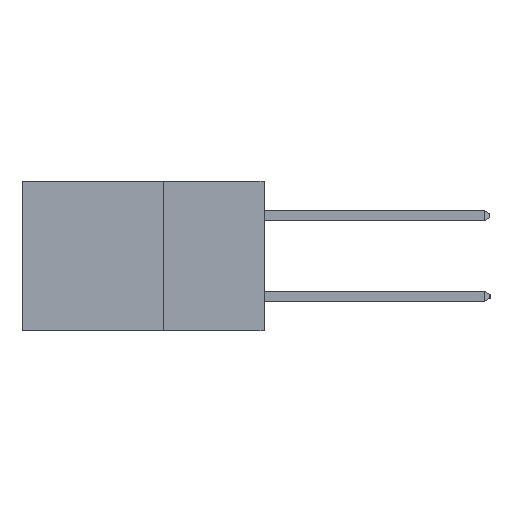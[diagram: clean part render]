
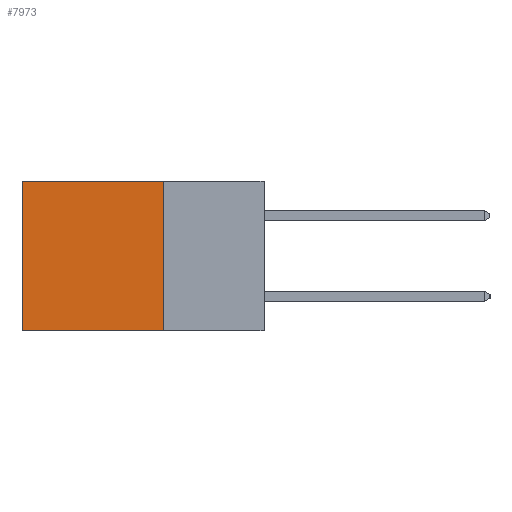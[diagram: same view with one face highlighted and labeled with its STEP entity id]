
A CAD part, left-side view. The second image highlights one B-rep face of the part: STEP entity #7973.
In plain terms, the highlighted planar face has unit normal (-1, 0, 0).
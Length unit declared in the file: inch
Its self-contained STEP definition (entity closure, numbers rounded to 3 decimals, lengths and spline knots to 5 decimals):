
#307 = DIRECTION ( 'NONE',  ( 0., 0., -1. ) ) ;
#421 = VERTEX_POINT ( 'NONE', #8219 ) ;
#480 = EDGE_CURVE ( 'NONE', #1061, #9470, #7824, .T. ) ;
#952 = ORIENTED_EDGE ( 'NONE', *, *, #1966, .F. ) ;
#1061 = VERTEX_POINT ( 'NONE', #4202 ) ;
#1216 = VECTOR ( 'NONE', #10153, 39.37008 ) ;
#1253 = CARTESIAN_POINT ( 'NONE',  ( 0.2615, 0.25, -0.37 ) ) ;
#1736 = VERTEX_POINT ( 'NONE', #5232 ) ;
#1966 = EDGE_CURVE ( 'NONE', #9470, #421, #9518, .T. ) ;
#2122 = DIRECTION ( 'NONE',  ( 1., 0., 0. ) ) ;
#3432 = VECTOR ( 'NONE', #5014, 39.37008 ) ;
#3439 = LINE ( 'NONE', #5659, #9298 ) ;
#3731 = VECTOR ( 'NONE', #307, 39.37008 ) ;
#4202 = CARTESIAN_POINT ( 'NONE',  ( 0.2615, 0.25, 0. ) ) ;
#4224 = CARTESIAN_POINT ( 'NONE',  ( 0.2615, 0.25, -0.37 ) ) ;
#4474 = CARTESIAN_POINT ( 'NONE',  ( 0.2615, 0.25, -0.37 ) ) ;
#5014 = DIRECTION ( 'NONE',  ( 0., 1., 0. ) ) ;
#5218 = EDGE_LOOP ( 'NONE', ( #5604, #952, #5614, #5483 ) ) ;
#5232 = CARTESIAN_POINT ( 'NONE',  ( 0.2615, 0.6, 0. ) ) ;
#5483 = ORIENTED_EDGE ( 'NONE', *, *, #8576, .T. ) ;
#5604 = ORIENTED_EDGE ( 'NONE', *, *, #5955, .T. ) ;
#5614 = ORIENTED_EDGE ( 'NONE', *, *, #480, .F. ) ;
#5639 = FACE_OUTER_BOUND ( 'NONE', #5218, .T. ) ;
#5659 = CARTESIAN_POINT ( 'NONE',  ( 0.2615, 0.25, 0. ) ) ;
#5955 = EDGE_CURVE ( 'NONE', #1736, #421, #9545, .T. ) ;
#6048 = PLANE ( 'NONE',  #9008 ) ;
#6607 = CARTESIAN_POINT ( 'NONE',  ( 0.2615, 0.25, -0.37 ) ) ;
#7548 = DIRECTION ( 'NONE',  ( 0., 0., -1. ) ) ;
#7824 = LINE ( 'NONE', #1253, #3731 ) ;
#7946 = CARTESIAN_POINT ( 'NONE',  ( 0.2615, 0.6, -0.37 ) ) ;
#7973 = ADVANCED_FACE ( 'NONE', ( #5639 ), #6048, .F. ) ;
#8219 = CARTESIAN_POINT ( 'NONE',  ( 0.2615, 0.6, -0.37 ) ) ;
#8576 = EDGE_CURVE ( 'NONE', #1061, #1736, #3439, .T. ) ;
#9008 = AXIS2_PLACEMENT_3D ( 'NONE', #4474, #2122, #7548 ) ;
#9298 = VECTOR ( 'NONE', #10159, 39.37008 ) ;
#9470 = VERTEX_POINT ( 'NONE', #6607 ) ;
#9518 = LINE ( 'NONE', #4224, #3432 ) ;
#9545 = LINE ( 'NONE', #7946, #1216 ) ;
#10153 = DIRECTION ( 'NONE',  ( 0., 0., -1. ) ) ;
#10159 = DIRECTION ( 'NONE',  ( 0., 1., 0. ) ) ;
